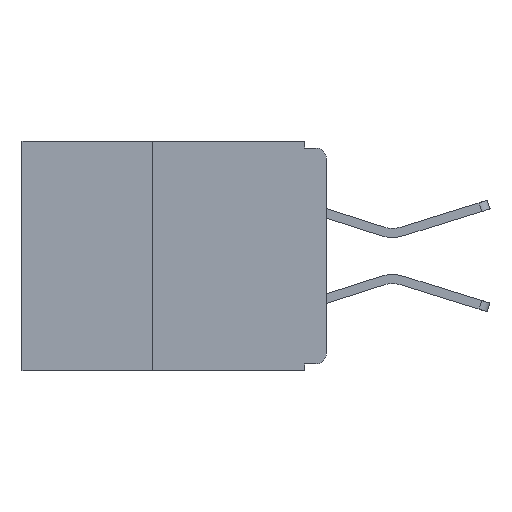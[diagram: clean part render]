
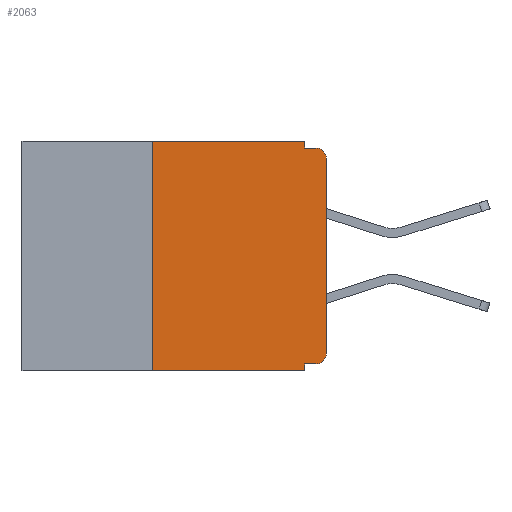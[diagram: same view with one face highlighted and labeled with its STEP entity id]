
A CAD part, left-side view. The second image highlights one B-rep face of the part: STEP entity #2063.
In plain terms, the highlighted planar face has unit normal (-1, 0, 0).
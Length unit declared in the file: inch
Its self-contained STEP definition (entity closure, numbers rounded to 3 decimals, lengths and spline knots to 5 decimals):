
#127 = CARTESIAN_POINT ( 'NONE',  ( 0., 0., -0.025 ) ) ;
#155 = AXIS2_PLACEMENT_3D ( 'NONE', #4557, #1168, #8999 ) ;
#526 = DIRECTION ( 'NONE',  ( 0., 0., 1. ) ) ;
#1168 = DIRECTION ( 'NONE',  ( 1., 0., 0. ) ) ;
#1275 = EDGE_CURVE ( 'NONE', #5116, #12469, #6748, .T. ) ;
#1317 = EDGE_LOOP ( 'NONE', ( #4241, #6977, #10375, #3835, #7256, #3879, #4723, #3746, #13108, #7699 ) ) ;
#1787 = CARTESIAN_POINT ( 'NONE',  ( 0., 0.015, -0.32 ) ) ;
#1937 = VERTEX_POINT ( 'NONE', #12050 ) ;
#2008 = LINE ( 'NONE', #6227, #5034 ) ;
#2063 = ADVANCED_FACE ( 'NONE', ( #2864 ), #12275, .F. ) ;
#2528 = VECTOR ( 'NONE', #4062, 39.37008 ) ;
#2638 = LINE ( 'NONE', #11746, #5660 ) ;
#2864 = FACE_OUTER_BOUND ( 'NONE', #1317, .T. ) ;
#3048 = VERTEX_POINT ( 'NONE', #9764 ) ;
#3072 = CARTESIAN_POINT ( 'NONE',  ( 0., 0.015, -0.01 ) ) ;
#3632 = CARTESIAN_POINT ( 'NONE',  ( 0., 0.437, -0.33 ) ) ;
#3746 = ORIENTED_EDGE ( 'NONE', *, *, #8337, .F. ) ;
#3835 = ORIENTED_EDGE ( 'NONE', *, *, #13684, .F. ) ;
#3879 = ORIENTED_EDGE ( 'NONE', *, *, #8881, .F. ) ;
#4062 = DIRECTION ( 'NONE',  ( 0., 1., 0. ) ) ;
#4102 = CARTESIAN_POINT ( 'NONE',  ( 0., 0.031, -0.32 ) ) ;
#4241 = ORIENTED_EDGE ( 'NONE', *, *, #9483, .T. ) ;
#4422 = EDGE_CURVE ( 'NONE', #12331, #12685, #12521, .T. ) ;
#4557 = CARTESIAN_POINT ( 'NONE',  ( 0., 0.437, 0. ) ) ;
#4723 = ORIENTED_EDGE ( 'NONE', *, *, #1275, .T. ) ;
#4890 = VECTOR ( 'NONE', #5990, 39.37008 ) ;
#4961 = DIRECTION ( 'NONE',  ( -1., 0., 0. ) ) ;
#4962 = CARTESIAN_POINT ( 'NONE',  ( 0., 0.015, -0.025 ) ) ;
#5034 = VECTOR ( 'NONE', #11723, 39.37008 ) ;
#5058 = CARTESIAN_POINT ( 'NONE',  ( 0., 0., 0. ) ) ;
#5116 = VERTEX_POINT ( 'NONE', #7407 ) ;
#5660 = VECTOR ( 'NONE', #12845, 39.37008 ) ;
#5949 = CARTESIAN_POINT ( 'NONE',  ( 0., 0.031, 0. ) ) ;
#5990 = DIRECTION ( 'NONE',  ( 0., -1., 0. ) ) ;
#6082 = DIRECTION ( 'NONE',  ( 0., 0., -1. ) ) ;
#6086 = VECTOR ( 'NONE', #7049, 39.37008 ) ;
#6089 = CARTESIAN_POINT ( 'NONE',  ( 0., 0.031, -0.33 ) ) ;
#6227 = CARTESIAN_POINT ( 'NONE',  ( 0., 0., -0.01 ) ) ;
#6350 = EDGE_CURVE ( 'NONE', #9399, #12685, #2008, .T. ) ;
#6748 = LINE ( 'NONE', #3632, #12276 ) ;
#6977 = ORIENTED_EDGE ( 'NONE', *, *, #4422, .T. ) ;
#7037 = VECTOR ( 'NONE', #14096, 39.37008 ) ;
#7049 = DIRECTION ( 'NONE',  ( 0., 0., -1. ) ) ;
#7081 = CARTESIAN_POINT ( 'NONE',  ( 0., 0.437, 0. ) ) ;
#7136 = CARTESIAN_POINT ( 'NONE',  ( 0., 0.031, -0.01 ) ) ;
#7188 = LINE ( 'NONE', #5058, #12707 ) ;
#7256 = ORIENTED_EDGE ( 'NONE', *, *, #12420, .F. ) ;
#7332 = CIRCLE ( 'NONE', #7536, 0.015 ) ;
#7407 = CARTESIAN_POINT ( 'NONE',  ( 0., 0.25, -0.33 ) ) ;
#7464 = CARTESIAN_POINT ( 'NONE',  ( 0., 0., -0.32 ) ) ;
#7475 = CARTESIAN_POINT ( 'NONE',  ( 0., 0.031, -0.33 ) ) ;
#7536 = AXIS2_PLACEMENT_3D ( 'NONE', #11577, #4961, #12672 ) ;
#7699 = ORIENTED_EDGE ( 'NONE', *, *, #11384, .T. ) ;
#7818 = LINE ( 'NONE', #7081, #4890 ) ;
#8337 = EDGE_CURVE ( 'NONE', #10426, #12469, #9997, .T. ) ;
#8411 = DIRECTION ( 'NONE',  ( 0., -1., 0. ) ) ;
#8573 = CARTESIAN_POINT ( 'NONE',  ( 0., 0.031, 0. ) ) ;
#8881 = EDGE_CURVE ( 'NONE', #5116, #3048, #2638, .T. ) ;
#8999 = DIRECTION ( 'NONE',  ( 0., 0., -1. ) ) ;
#9016 = LINE ( 'NONE', #5949, #6086 ) ;
#9399 = VERTEX_POINT ( 'NONE', #7136 ) ;
#9483 = EDGE_CURVE ( 'NONE', #1937, #12331, #7188, .T. ) ;
#9504 = AXIS2_PLACEMENT_3D ( 'NONE', #4962, #12675, #6082 ) ;
#9764 = CARTESIAN_POINT ( 'NONE',  ( 0., 0.25, 0. ) ) ;
#9997 = LINE ( 'NONE', #7475, #7037 ) ;
#10375 = ORIENTED_EDGE ( 'NONE', *, *, #6350, .F. ) ;
#10426 = VERTEX_POINT ( 'NONE', #4102 ) ;
#11064 = VERTEX_POINT ( 'NONE', #1787 ) ;
#11384 = EDGE_CURVE ( 'NONE', #11064, #1937, #7332, .T. ) ;
#11577 = CARTESIAN_POINT ( 'NONE',  ( 0., 0.015, -0.305 ) ) ;
#11723 = DIRECTION ( 'NONE',  ( 0., -1., 0. ) ) ;
#11746 = CARTESIAN_POINT ( 'NONE',  ( 0., 0.25, -0.33 ) ) ;
#12050 = CARTESIAN_POINT ( 'NONE',  ( 0., 0., -0.305 ) ) ;
#12275 = PLANE ( 'NONE',  #155 ) ;
#12276 = VECTOR ( 'NONE', #8411, 39.37008 ) ;
#12331 = VERTEX_POINT ( 'NONE', #127 ) ;
#12420 = EDGE_CURVE ( 'NONE', #3048, #13823, #7818, .T. ) ;
#12469 = VERTEX_POINT ( 'NONE', #6089 ) ;
#12521 = CIRCLE ( 'NONE', #9504, 0.015 ) ;
#12672 = DIRECTION ( 'NONE',  ( 0., 0., -1. ) ) ;
#12675 = DIRECTION ( 'NONE',  ( -1., 0., 0. ) ) ;
#12685 = VERTEX_POINT ( 'NONE', #3072 ) ;
#12707 = VECTOR ( 'NONE', #526, 39.37008 ) ;
#12845 = DIRECTION ( 'NONE',  ( 0., 0., 1. ) ) ;
#13108 = ORIENTED_EDGE ( 'NONE', *, *, #13267, .F. ) ;
#13267 = EDGE_CURVE ( 'NONE', #11064, #10426, #14350, .T. ) ;
#13684 = EDGE_CURVE ( 'NONE', #13823, #9399, #9016, .T. ) ;
#13823 = VERTEX_POINT ( 'NONE', #8573 ) ;
#14096 = DIRECTION ( 'NONE',  ( 0., 0., -1. ) ) ;
#14350 = LINE ( 'NONE', #7464, #2528 ) ;
